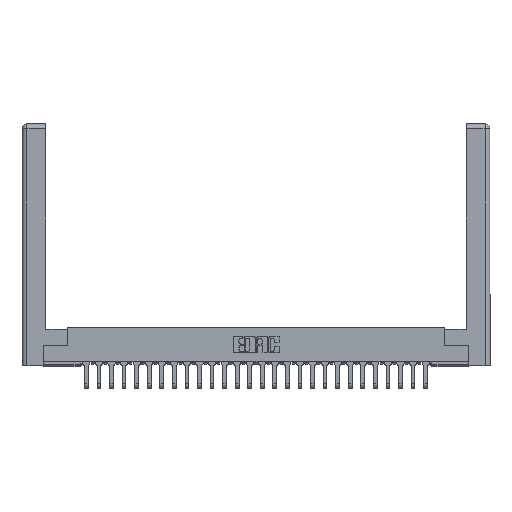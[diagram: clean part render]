
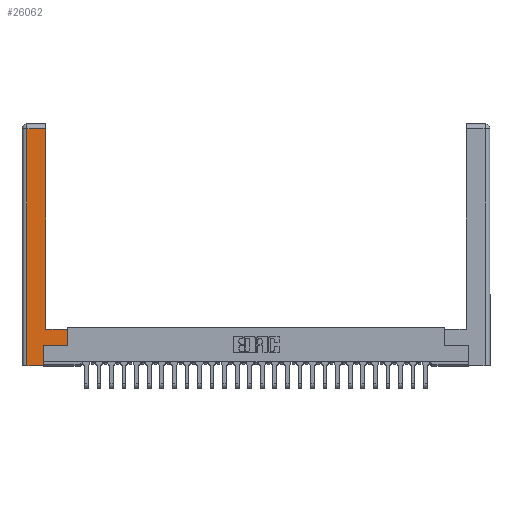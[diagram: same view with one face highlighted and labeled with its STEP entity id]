
A CAD part, top view. The second image highlights one B-rep face of the part: STEP entity #26062.
In plain terms, the highlighted planar face has unit normal (0, 0, 1).
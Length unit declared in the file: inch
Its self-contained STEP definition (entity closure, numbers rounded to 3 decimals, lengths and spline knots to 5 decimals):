
#65 = VECTOR ( 'NONE', #24844, 39.37008 ) ;
#198 = EDGE_CURVE ( 'NONE', #23286, #18756, #1652, .T. ) ;
#525 = CARTESIAN_POINT ( 'NONE',  ( 0.265, 0., 0. ) ) ;
#825 = DIRECTION ( 'NONE',  ( 0., 1., 0. ) ) ;
#912 = CARTESIAN_POINT ( 'NONE',  ( 0.265, 0., 0. ) ) ;
#921 = DIRECTION ( 'NONE',  ( 0., 1., 0. ) ) ;
#1588 = EDGE_CURVE ( 'NONE', #25741, #20900, #12702, .T. ) ;
#1652 = LINE ( 'NONE', #22969, #13415 ) ;
#3065 = CARTESIAN_POINT ( 'NONE',  ( 0.565, 0.45, 0. ) ) ;
#3921 = VECTOR ( 'NONE', #7335, 39.37008 ) ;
#5162 = EDGE_CURVE ( 'NONE', #20900, #25614, #8296, .T. ) ;
#5867 = CARTESIAN_POINT ( 'NONE',  ( 0.0615, 0., 0. ) ) ;
#6390 = VECTOR ( 'NONE', #29136, 39.37008 ) ;
#6899 = AXIS2_PLACEMENT_3D ( 'NONE', #13437, #13604, #22625 ) ;
#7335 = DIRECTION ( 'NONE',  ( 0., 1., 0. ) ) ;
#7557 = DIRECTION ( 'NONE',  ( -1., 0., 0. ) ) ;
#7949 = EDGE_CURVE ( 'NONE', #8938, #12422, #17896, .T. ) ;
#8296 = LINE ( 'NONE', #525, #6390 ) ;
#8779 = FACE_OUTER_BOUND ( 'NONE', #21427, .T. ) ;
#8938 = VERTEX_POINT ( 'NONE', #3065 ) ;
#8974 = DIRECTION ( 'NONE',  ( 1., 0., 0. ) ) ;
#9647 = VECTOR ( 'NONE', #921, 39.37008 ) ;
#10050 = LINE ( 'NONE', #28852, #18807 ) ;
#10075 = ORIENTED_EDGE ( 'NONE', *, *, #20383, .T. ) ;
#10586 = CARTESIAN_POINT ( 'NONE',  ( 0.295, 0.45, 0. ) ) ;
#11998 = VECTOR ( 'NONE', #825, 39.37008 ) ;
#12422 = VERTEX_POINT ( 'NONE', #23400 ) ;
#12651 = LINE ( 'NONE', #22140, #11998 ) ;
#12702 = LINE ( 'NONE', #27182, #65 ) ;
#13114 = CARTESIAN_POINT ( 'NONE',  ( 0.295, 2.94, 0. ) ) ;
#13233 = EDGE_CURVE ( 'NONE', #15807, #25741, #10050, .T. ) ;
#13415 = VECTOR ( 'NONE', #8974, 39.37008 ) ;
#13437 = CARTESIAN_POINT ( 'NONE',  ( 0., 0., 0. ) ) ;
#13475 = VECTOR ( 'NONE', #27229, 39.37008 ) ;
#13604 = DIRECTION ( 'NONE',  ( 0., 0., -1. ) ) ;
#13830 = CARTESIAN_POINT ( 'NONE',  ( 0.0615, 2.94, 0. ) ) ;
#14368 = ORIENTED_EDGE ( 'NONE', *, *, #13233, .T. ) ;
#15807 = VERTEX_POINT ( 'NONE', #13114 ) ;
#17896 = LINE ( 'NONE', #10586, #13475 ) ;
#18427 = ORIENTED_EDGE ( 'NONE', *, *, #1588, .T. ) ;
#18756 = VERTEX_POINT ( 'NONE', #26134 ) ;
#18807 = VECTOR ( 'NONE', #7557, 39.37008 ) ;
#20053 = ORIENTED_EDGE ( 'NONE', *, *, #30585, .T. ) ;
#20383 = EDGE_CURVE ( 'NONE', #12422, #15807, #26609, .T. ) ;
#20900 = VERTEX_POINT ( 'NONE', #5867 ) ;
#21399 = ORIENTED_EDGE ( 'NONE', *, *, #7949, .T. ) ;
#21427 = EDGE_LOOP ( 'NONE', ( #10075, #14368, #18427, #29904, #23155, #23194, #20053, #21399 ) ) ;
#21941 = LINE ( 'NONE', #24270, #3921 ) ;
#22140 = CARTESIAN_POINT ( 'NONE',  ( 0.565, 0.45, 0. ) ) ;
#22625 = DIRECTION ( 'NONE',  ( -1., 0., 0. ) ) ;
#22969 = CARTESIAN_POINT ( 'NONE',  ( 0.565, 0.245, 0. ) ) ;
#23155 = ORIENTED_EDGE ( 'NONE', *, *, #26352, .T. ) ;
#23194 = ORIENTED_EDGE ( 'NONE', *, *, #198, .T. ) ;
#23286 = VERTEX_POINT ( 'NONE', #23878 ) ;
#23400 = CARTESIAN_POINT ( 'NONE',  ( 0.295, 0.45, 0. ) ) ;
#23878 = CARTESIAN_POINT ( 'NONE',  ( 0.265, 0.245, 0. ) ) ;
#24270 = CARTESIAN_POINT ( 'NONE',  ( 0.265, 0.245, 0. ) ) ;
#24844 = DIRECTION ( 'NONE',  ( 0., -1., 0. ) ) ;
#25614 = VERTEX_POINT ( 'NONE', #912 ) ;
#25741 = VERTEX_POINT ( 'NONE', #13830 ) ;
#26062 = ADVANCED_FACE ( 'NONE', ( #8779 ), #27293, .F. ) ;
#26134 = CARTESIAN_POINT ( 'NONE',  ( 0.565, 0.245, 0. ) ) ;
#26352 = EDGE_CURVE ( 'NONE', #25614, #23286, #21941, .T. ) ;
#26609 = LINE ( 'NONE', #29234, #9647 ) ;
#27182 = CARTESIAN_POINT ( 'NONE',  ( 0.0615, 0., 0. ) ) ;
#27229 = DIRECTION ( 'NONE',  ( -1., 0., 0. ) ) ;
#27293 = PLANE ( 'NONE',  #6899 ) ;
#28852 = CARTESIAN_POINT ( 'NONE',  ( 0.0615, 2.94, 0. ) ) ;
#29136 = DIRECTION ( 'NONE',  ( 1., 0., 0. ) ) ;
#29234 = CARTESIAN_POINT ( 'NONE',  ( 0.295, 3., 0. ) ) ;
#29904 = ORIENTED_EDGE ( 'NONE', *, *, #5162, .T. ) ;
#30585 = EDGE_CURVE ( 'NONE', #18756, #8938, #12651, .T. ) ;
